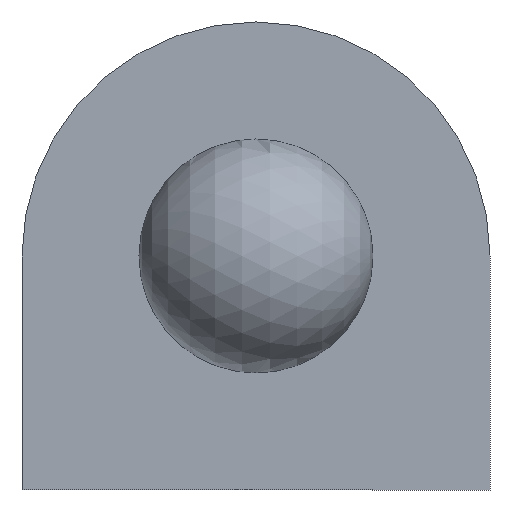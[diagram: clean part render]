
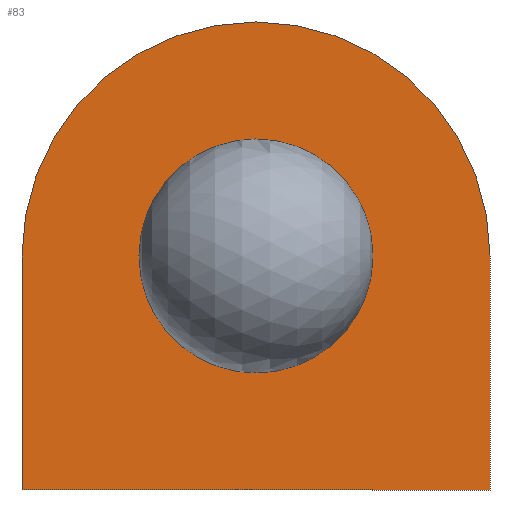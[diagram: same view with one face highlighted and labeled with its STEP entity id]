
A CAD part, left-side view. The second image highlights one B-rep face of the part: STEP entity #83.
In plain terms, the highlighted planar face has unit normal (-1, 0, 0).
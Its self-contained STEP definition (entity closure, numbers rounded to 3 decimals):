
#1 = DIRECTION ( 'NONE',  ( -1., 0., 0. ) ) ;
#6 = DIRECTION ( 'NONE',  ( -1., 0., 0. ) ) ;
#9 = DIRECTION ( 'NONE',  ( 1., 0., 0. ) ) ;
#18 = CIRCLE ( 'NONE', #166, 5. ) ;
#20 = VECTOR ( 'NONE', #28, 1000. ) ;
#24 = LINE ( 'NONE', #204, #20 ) ;
#25 = VECTOR ( 'NONE', #216, 1000. ) ;
#28 = DIRECTION ( 'NONE',  ( 0., -1., 0. ) ) ;
#29 = VECTOR ( 'NONE', #285, 1000. ) ;
#31 = LINE ( 'NONE', #104, #29 ) ;
#34 = CIRCLE ( 'NONE', #173, 5. ) ;
#35 = LINE ( 'NONE', #109, #25 ) ;
#36 = CIRCLE ( 'NONE', #178, 2.5 ) ;
#39 = CIRCLE ( 'NONE', #174, 2.5 ) ;
#66 = ORIENTED_EDGE ( 'NONE', *, *, #254, .F. ) ;
#83 = ADVANCED_FACE ( 'NONE', ( #239, #187 ), #201, .F. ) ;
#84 = DIRECTION ( 'NONE',  ( 0., 0., -1. ) ) ;
#86 = CARTESIAN_POINT ( 'NONE',  ( 0., 0., 0. ) ) ;
#103 = DIRECTION ( 'NONE',  ( 1., 0., 0. ) ) ;
#104 = CARTESIAN_POINT ( 'NONE',  ( 0., -5., 0. ) ) ;
#109 = CARTESIAN_POINT ( 'NONE',  ( 0., 5., 0. ) ) ;
#111 = CARTESIAN_POINT ( 'NONE',  ( 0., 0., 0. ) ) ;
#113 = DIRECTION ( 'NONE',  ( 0., 0., -1. ) ) ;
#120 = CARTESIAN_POINT ( 'NONE',  ( 0., -5., 0. ) ) ;
#124 = CARTESIAN_POINT ( 'NONE',  ( 0., 0., 0. ) ) ;
#131 = CARTESIAN_POINT ( 'NONE',  ( 0., 0., 0. ) ) ;
#132 = CARTESIAN_POINT ( 'NONE',  ( 0., -5., -5. ) ) ;
#134 = VERTEX_POINT ( 'NONE', #132 ) ;
#137 = EDGE_LOOP ( 'NONE', ( #156, #260, #268, #276, #159 ) ) ;
#150 = VERTEX_POINT ( 'NONE', #215 ) ;
#156 = ORIENTED_EDGE ( 'NONE', *, *, #278, .T. ) ;
#159 = ORIENTED_EDGE ( 'NONE', *, *, #263, .F. ) ;
#160 = VERTEX_POINT ( 'NONE', #266 ) ;
#166 = AXIS2_PLACEMENT_3D ( 'NONE', #221, #103, #208 ) ;
#168 = CARTESIAN_POINT ( 'NONE',  ( 0., 0., 5. ) ) ;
#173 = AXIS2_PLACEMENT_3D ( 'NONE', #86, #9, #307 ) ;
#174 = AXIS2_PLACEMENT_3D ( 'NONE', #131, #1, #113 ) ;
#178 = AXIS2_PLACEMENT_3D ( 'NONE', #111, #6, #84 ) ;
#186 = VERTEX_POINT ( 'NONE', #120 ) ;
#187 = FACE_BOUND ( 'NONE', #312, .T. ) ;
#192 = DIRECTION ( 'NONE',  ( 1., 0., 0. ) ) ;
#201 = PLANE ( 'NONE',  #206 ) ;
#204 = CARTESIAN_POINT ( 'NONE',  ( 0., 0., -5. ) ) ;
#206 = AXIS2_PLACEMENT_3D ( 'NONE', #124, #192, #274 ) ;
#208 = DIRECTION ( 'NONE',  ( 0., 0., -1. ) ) ;
#215 = CARTESIAN_POINT ( 'NONE',  ( 0., 0., 2.5 ) ) ;
#216 = DIRECTION ( 'NONE',  ( 0., 0., -1. ) ) ;
#221 = CARTESIAN_POINT ( 'NONE',  ( 0., 0., 0. ) ) ;
#239 = FACE_OUTER_BOUND ( 'NONE', #137, .T. ) ;
#253 = VERTEX_POINT ( 'NONE', #168 ) ;
#254 = EDGE_CURVE ( 'NONE', #150, #310, #39, .T. ) ;
#257 = EDGE_CURVE ( 'NONE', #310, #150, #36, .T. ) ;
#260 = ORIENTED_EDGE ( 'NONE', *, *, #272, .T. ) ;
#261 = VERTEX_POINT ( 'NONE', #290 ) ;
#263 = EDGE_CURVE ( 'NONE', #261, #253, #34, .T. ) ;
#266 = CARTESIAN_POINT ( 'NONE',  ( 0., 5., -5. ) ) ;
#267 = EDGE_CURVE ( 'NONE', #186, #134, #31, .T. ) ;
#268 = ORIENTED_EDGE ( 'NONE', *, *, #267, .F. ) ;
#272 = EDGE_CURVE ( 'NONE', #160, #134, #24, .T. ) ;
#274 = DIRECTION ( 'NONE',  ( 0., 0., -1. ) ) ;
#276 = ORIENTED_EDGE ( 'NONE', *, *, #288, .F. ) ;
#278 = EDGE_CURVE ( 'NONE', #261, #160, #35, .T. ) ;
#285 = DIRECTION ( 'NONE',  ( 0., 0., -1. ) ) ;
#288 = EDGE_CURVE ( 'NONE', #253, #186, #18, .T. ) ;
#290 = CARTESIAN_POINT ( 'NONE',  ( 0., 5., 0. ) ) ;
#291 = ORIENTED_EDGE ( 'NONE', *, *, #257, .F. ) ;
#305 = CARTESIAN_POINT ( 'NONE',  ( 0., 0., -2.5 ) ) ;
#307 = DIRECTION ( 'NONE',  ( 0., 0., -1. ) ) ;
#310 = VERTEX_POINT ( 'NONE', #305 ) ;
#312 = EDGE_LOOP ( 'NONE', ( #291, #66 ) ) ;
